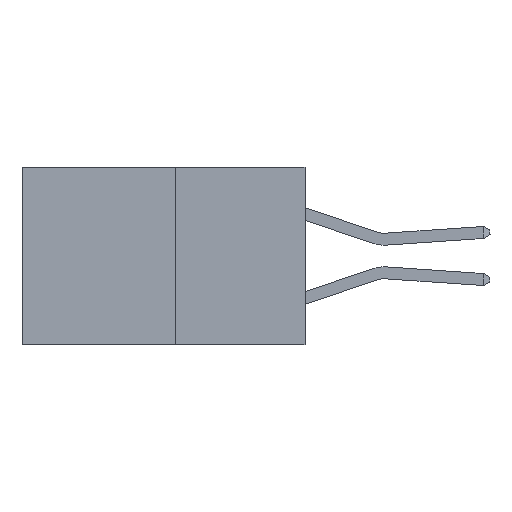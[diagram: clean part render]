
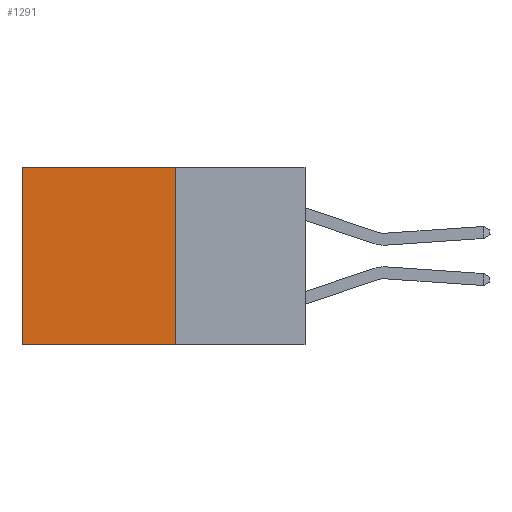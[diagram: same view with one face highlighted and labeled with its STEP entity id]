
A CAD part, left-side view. The second image highlights one B-rep face of the part: STEP entity #1291.
In plain terms, the highlighted planar face has unit normal (-1, 0, 0).
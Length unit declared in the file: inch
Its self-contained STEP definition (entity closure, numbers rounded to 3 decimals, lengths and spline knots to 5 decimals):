
#211 = CARTESIAN_POINT ( 'NONE',  ( 0.277, 0.59, -0.37 ) ) ;
#409 = CARTESIAN_POINT ( 'NONE',  ( 0.277, 0.59, 0. ) ) ;
#648 = LINE ( 'NONE', #2906, #4806 ) ;
#771 = CARTESIAN_POINT ( 'NONE',  ( 0.277, 0.27, -0.37 ) ) ;
#1031 = VECTOR ( 'NONE', #1102, 39.37008 ) ;
#1102 = DIRECTION ( 'NONE',  ( 0., 0., -1. ) ) ;
#1227 = EDGE_CURVE ( 'NONE', #7477, #7425, #9980, .T. ) ;
#1291 = ADVANCED_FACE ( 'NONE', ( #9492 ), #7804, .F. ) ;
#1305 = DIRECTION ( 'NONE',  ( 0., 1., 0. ) ) ;
#1817 = EDGE_CURVE ( 'NONE', #7425, #7680, #6778, .T. ) ;
#1859 = DIRECTION ( 'NONE',  ( 0., 1., 0. ) ) ;
#2157 = ORIENTED_EDGE ( 'NONE', *, *, #2243, .T. ) ;
#2243 = EDGE_CURVE ( 'NONE', #7477, #8967, #648, .T. ) ;
#2293 = CARTESIAN_POINT ( 'NONE',  ( 0.277, 0.27, -0.37 ) ) ;
#2547 = CARTESIAN_POINT ( 'NONE',  ( 0.277, 0.27, 0. ) ) ;
#2628 = DIRECTION ( 'NONE',  ( 0., 0., -1. ) ) ;
#2906 = CARTESIAN_POINT ( 'NONE',  ( 0.277, 0.27, 0. ) ) ;
#3263 = ORIENTED_EDGE ( 'NONE', *, *, #1817, .F. ) ;
#4413 = CARTESIAN_POINT ( 'NONE',  ( 0.277, 0.59, -0.37 ) ) ;
#4697 = ORIENTED_EDGE ( 'NONE', *, *, #8318, .T. ) ;
#4806 = VECTOR ( 'NONE', #1859, 39.37008 ) ;
#5265 = CARTESIAN_POINT ( 'NONE',  ( 0.277, 0.27, -0.37 ) ) ;
#5604 = ORIENTED_EDGE ( 'NONE', *, *, #1227, .F. ) ;
#6778 = LINE ( 'NONE', #9031, #7299 ) ;
#7299 = VECTOR ( 'NONE', #1305, 39.37008 ) ;
#7425 = VERTEX_POINT ( 'NONE', #771 ) ;
#7477 = VERTEX_POINT ( 'NONE', #2547 ) ;
#7653 = LINE ( 'NONE', #211, #1031 ) ;
#7667 = DIRECTION ( 'NONE',  ( 1., 0., 0. ) ) ;
#7680 = VERTEX_POINT ( 'NONE', #4413 ) ;
#7804 = PLANE ( 'NONE',  #9743 ) ;
#7831 = VECTOR ( 'NONE', #2628, 39.37008 ) ;
#8318 = EDGE_CURVE ( 'NONE', #8967, #7680, #7653, .T. ) ;
#8847 = DIRECTION ( 'NONE',  ( 0., 0., -1. ) ) ;
#8967 = VERTEX_POINT ( 'NONE', #409 ) ;
#9031 = CARTESIAN_POINT ( 'NONE',  ( 0.277, 0.27, -0.37 ) ) ;
#9492 = FACE_OUTER_BOUND ( 'NONE', #10630, .T. ) ;
#9743 = AXIS2_PLACEMENT_3D ( 'NONE', #2293, #7667, #8847 ) ;
#9980 = LINE ( 'NONE', #5265, #7831 ) ;
#10630 = EDGE_LOOP ( 'NONE', ( #4697, #3263, #5604, #2157 ) ) ;
